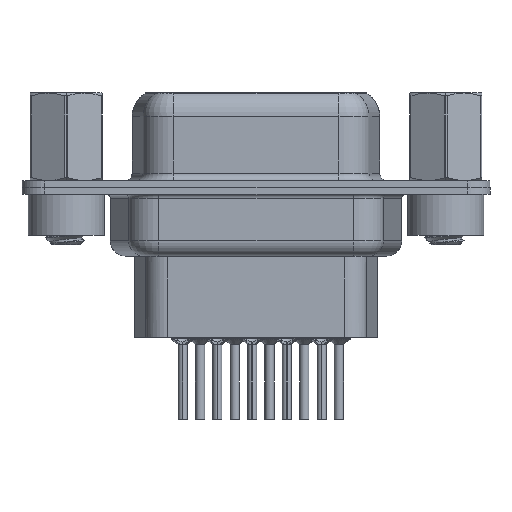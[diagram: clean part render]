
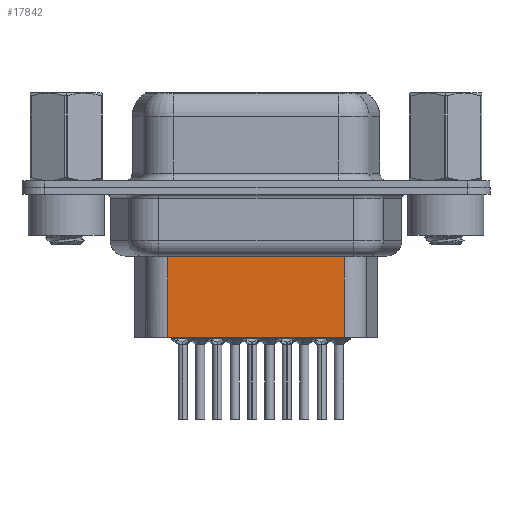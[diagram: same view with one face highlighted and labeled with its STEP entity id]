
A CAD part, front view. The second image highlights one B-rep face of the part: STEP entity #17842.
In plain terms, the highlighted planar face has unit normal (0, -1, 0).
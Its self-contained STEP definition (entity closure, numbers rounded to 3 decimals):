
#561 = CARTESIAN_POINT ( 'NONE',  ( 6.701, -3.5, -3.1 ) ) ;
#691 = VECTOR ( 'NONE', #13956, 1000. ) ;
#1011 = CARTESIAN_POINT ( 'NONE',  ( 6.701, -3.5, -9.85 ) ) ;
#2075 = LINE ( 'NONE', #17665, #28548 ) ;
#3126 = DIRECTION ( 'NONE',  ( 1., 0., 0. ) ) ;
#3525 = CARTESIAN_POINT ( 'NONE',  ( 18.289, -3.5, -3.1 ) ) ;
#4048 = ORIENTED_EDGE ( 'NONE', *, *, #25776, .F. ) ;
#4689 = VERTEX_POINT ( 'NONE', #1011 ) ;
#4963 = CARTESIAN_POINT ( 'NONE',  ( 18.289, -3.5, -9.85 ) ) ;
#7503 = EDGE_LOOP ( 'NONE', ( #8984, #21381, #8959, #4048 ) ) ;
#8237 = EDGE_CURVE ( 'NONE', #28024, #4689, #2075, .T. ) ;
#8959 = ORIENTED_EDGE ( 'NONE', *, *, #8237, .T. ) ;
#8984 = ORIENTED_EDGE ( 'NONE', *, *, #16350, .F. ) ;
#9548 = CARTESIAN_POINT ( 'NONE',  ( 6.701, -3.5, -9.85 ) ) ;
#13956 = DIRECTION ( 'NONE',  ( -1., 0., 0. ) ) ;
#14689 = DIRECTION ( 'NONE',  ( -1., 0., 0. ) ) ;
#14882 = VERTEX_POINT ( 'NONE', #4963 ) ;
#15973 = PLANE ( 'NONE',  #16364 ) ;
#16014 = VECTOR ( 'NONE', #18927, 1000. ) ;
#16350 = EDGE_CURVE ( 'NONE', #22840, #14882, #22769, .T. ) ;
#16364 = AXIS2_PLACEMENT_3D ( 'NONE', #561, #18529, #3126 ) ;
#17665 = CARTESIAN_POINT ( 'NONE',  ( 6.701, -3.5, -3.1 ) ) ;
#17842 = ADVANCED_FACE ( 'NONE', ( #23554 ), #15973, .T. ) ;
#18253 = CARTESIAN_POINT ( 'NONE',  ( 18.289, -3.5, -4.097 ) ) ;
#18529 = DIRECTION ( 'NONE',  ( 0., -1., 0. ) ) ;
#18927 = DIRECTION ( 'NONE',  ( 0., 0., -1. ) ) ;
#21381 = ORIENTED_EDGE ( 'NONE', *, *, #31536, .T. ) ;
#21716 = CARTESIAN_POINT ( 'NONE',  ( 6.701, -3.5, -4.097 ) ) ;
#22769 = LINE ( 'NONE', #3525, #16014 ) ;
#22840 = VERTEX_POINT ( 'NONE', #18253 ) ;
#23554 = FACE_OUTER_BOUND ( 'NONE', #7503, .T. ) ;
#25502 = VECTOR ( 'NONE', #14689, 1000. ) ;
#25776 = EDGE_CURVE ( 'NONE', #14882, #4689, #33050, .T. ) ;
#27931 = LINE ( 'NONE', #31745, #691 ) ;
#28019 = DIRECTION ( 'NONE',  ( 0., 0., -1. ) ) ;
#28024 = VERTEX_POINT ( 'NONE', #21716 ) ;
#28548 = VECTOR ( 'NONE', #28019, 1000. ) ;
#31536 = EDGE_CURVE ( 'NONE', #22840, #28024, #27931, .T. ) ;
#31745 = CARTESIAN_POINT ( 'NONE',  ( 6.454, -3.5, -4.097 ) ) ;
#33050 = LINE ( 'NONE', #9548, #25502 ) ;
